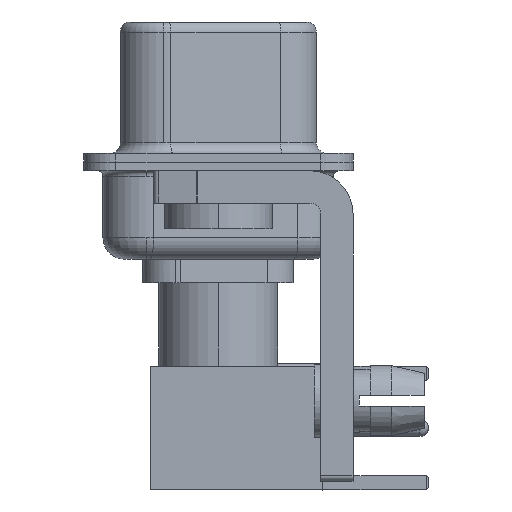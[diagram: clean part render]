
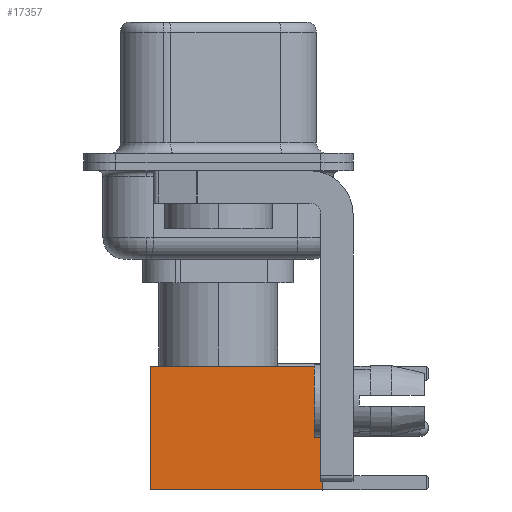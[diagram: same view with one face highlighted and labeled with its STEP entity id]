
A CAD part, left-side view. The second image highlights one B-rep face of the part: STEP entity #17357.
In plain terms, the highlighted face is planar.
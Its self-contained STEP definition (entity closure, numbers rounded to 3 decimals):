
#494 = CARTESIAN_POINT ( 'NONE',  ( 2.875, 2.875, 8. ) ) ;
#553 = EDGE_LOOP ( 'NONE', ( #18419, #26178, #1825, #1973 ) ) ;
#998 = VERTEX_POINT ( 'NONE', #9324 ) ;
#1470 = LINE ( 'NONE', #25696, #6442 ) ;
#1477 = CARTESIAN_POINT ( 'NONE',  ( 2.875, 2.875, 0. ) ) ;
#1825 = ORIENTED_EDGE ( 'NONE', *, *, #25973, .F. ) ;
#1973 = ORIENTED_EDGE ( 'NONE', *, *, #9812, .F. ) ;
#3778 = LINE ( 'NONE', #18372, #21136 ) ;
#5399 = DIRECTION ( 'NONE',  ( -1., 0., 0. ) ) ;
#6143 = DIRECTION ( 'NONE',  ( 0., 1., 0. ) ) ;
#6442 = VECTOR ( 'NONE', #20566, 1000. ) ;
#6675 = VERTEX_POINT ( 'NONE', #14968 ) ;
#9064 = DIRECTION ( 'NONE',  ( 0., 0., -1. ) ) ;
#9324 = CARTESIAN_POINT ( 'NONE',  ( -2.875, 2.875, 8. ) ) ;
#9812 = EDGE_CURVE ( 'NONE', #13870, #998, #1470, .T. ) ;
#12432 = AXIS2_PLACEMENT_3D ( 'NONE', #1477, #6143, #26821 ) ;
#12642 = CARTESIAN_POINT ( 'NONE',  ( -2.875, 2.875, 0. ) ) ;
#13269 = FACE_OUTER_BOUND ( 'NONE', #553, .T. ) ;
#13870 = VERTEX_POINT ( 'NONE', #494 ) ;
#14125 = VECTOR ( 'NONE', #9064, 1000. ) ;
#14388 = CARTESIAN_POINT ( 'NONE',  ( 0., 2.875, 0. ) ) ;
#14726 = EDGE_CURVE ( 'NONE', #6675, #28060, #17354, .T. ) ;
#14968 = CARTESIAN_POINT ( 'NONE',  ( 2.875, 2.875, 0. ) ) ;
#17354 = LINE ( 'NONE', #14388, #29309 ) ;
#17357 = ADVANCED_FACE ( 'NONE', ( #13269 ), #22775, .T. ) ;
#18214 = DIRECTION ( 'NONE',  ( 0., 0., -1. ) ) ;
#18372 = CARTESIAN_POINT ( 'NONE',  ( -2.875, 2.875, 0. ) ) ;
#18419 = ORIENTED_EDGE ( 'NONE', *, *, #25547, .T. ) ;
#20566 = DIRECTION ( 'NONE',  ( -1., 0., 0. ) ) ;
#21136 = VECTOR ( 'NONE', #18214, 1000. ) ;
#22775 = PLANE ( 'NONE',  #12432 ) ;
#25547 = EDGE_CURVE ( 'NONE', #13870, #6675, #30089, .T. ) ;
#25696 = CARTESIAN_POINT ( 'NONE',  ( 0., 2.875, 8. ) ) ;
#25973 = EDGE_CURVE ( 'NONE', #998, #28060, #3778, .T. ) ;
#26178 = ORIENTED_EDGE ( 'NONE', *, *, #14726, .T. ) ;
#26821 = DIRECTION ( 'NONE',  ( 0., 0., 1. ) ) ;
#28060 = VERTEX_POINT ( 'NONE', #12642 ) ;
#29309 = VECTOR ( 'NONE', #5399, 1000. ) ;
#30089 = LINE ( 'NONE', #30395, #14125 ) ;
#30395 = CARTESIAN_POINT ( 'NONE',  ( 2.875, 2.875, 0. ) ) ;
